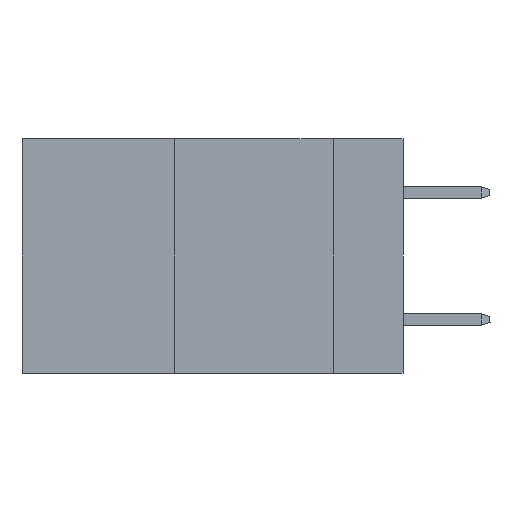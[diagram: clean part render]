
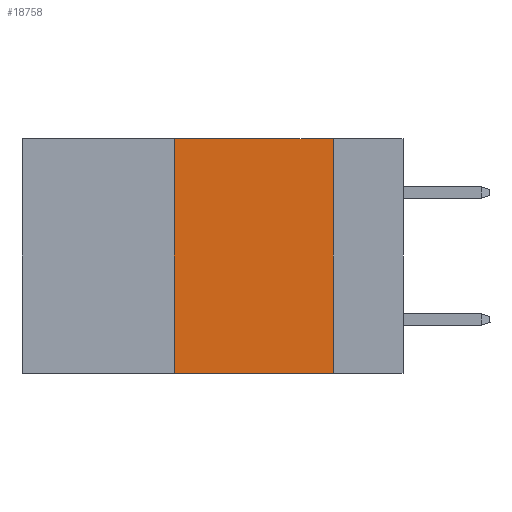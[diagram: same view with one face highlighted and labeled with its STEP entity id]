
A CAD part, left-side view. The second image highlights one B-rep face of the part: STEP entity #18758.
In plain terms, the highlighted planar face has unit normal (-1, 0, 0).
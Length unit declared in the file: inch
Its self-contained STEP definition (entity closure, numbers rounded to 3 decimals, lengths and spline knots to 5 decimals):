
#2084 = VERTEX_POINT ( 'NONE', #18589 ) ;
#2657 = LINE ( 'NONE', #15431, #31532 ) ;
#2737 = VERTEX_POINT ( 'NONE', #8233 ) ;
#3183 = DIRECTION ( 'NONE',  ( 0., 0., -1. ) ) ;
#3955 = DIRECTION ( 'NONE',  ( 0., -1., 0. ) ) ;
#4764 = AXIS2_PLACEMENT_3D ( 'NONE', #30969, #25291, #20306 ) ;
#8233 = CARTESIAN_POINT ( 'NONE',  ( 0., 0.36, 0. ) ) ;
#8951 = VECTOR ( 'NONE', #9687, 39.37008 ) ;
#8992 = CARTESIAN_POINT ( 'NONE',  ( 0., 0.36, -0.37 ) ) ;
#9687 = DIRECTION ( 'NONE',  ( 0., -1., 0. ) ) ;
#9983 = VECTOR ( 'NONE', #3183, 39.37008 ) ;
#10035 = FACE_OUTER_BOUND ( 'NONE', #23592, .T. ) ;
#12499 = ORIENTED_EDGE ( 'NONE', *, *, #22464, .F. ) ;
#12873 = DIRECTION ( 'NONE',  ( 0., 0., 1. ) ) ;
#13280 = ORIENTED_EDGE ( 'NONE', *, *, #28120, .F. ) ;
#15431 = CARTESIAN_POINT ( 'NONE',  ( 0., 0.36, 0. ) ) ;
#16124 = LINE ( 'NONE', #26617, #9983 ) ;
#16778 = LINE ( 'NONE', #27406, #31529 ) ;
#16931 = ORIENTED_EDGE ( 'NONE', *, *, #25445, .T. ) ;
#18466 = EDGE_CURVE ( 'NONE', #33410, #2737, #2657, .T. ) ;
#18589 = CARTESIAN_POINT ( 'NONE',  ( 0., 0.11, 0. ) ) ;
#18758 = ADVANCED_FACE ( 'NONE', ( #10035 ), #22745, .F. ) ;
#20306 = DIRECTION ( 'NONE',  ( 0., 0., -1. ) ) ;
#20839 = CARTESIAN_POINT ( 'NONE',  ( 0., 0.11, -0.37 ) ) ;
#21316 = VERTEX_POINT ( 'NONE', #20839 ) ;
#22464 = EDGE_CURVE ( 'NONE', #2084, #21316, #16124, .T. ) ;
#22715 = LINE ( 'NONE', #33177, #8951 ) ;
#22745 = PLANE ( 'NONE',  #4764 ) ;
#23592 = EDGE_LOOP ( 'NONE', ( #12499, #13280, #27113, #16931 ) ) ;
#25291 = DIRECTION ( 'NONE',  ( 1., 0., 0. ) ) ;
#25445 = EDGE_CURVE ( 'NONE', #33410, #21316, #22715, .T. ) ;
#26617 = CARTESIAN_POINT ( 'NONE',  ( 0., 0.11, 0. ) ) ;
#27113 = ORIENTED_EDGE ( 'NONE', *, *, #18466, .F. ) ;
#27406 = CARTESIAN_POINT ( 'NONE',  ( 0., 0.6, 0. ) ) ;
#28120 = EDGE_CURVE ( 'NONE', #2737, #2084, #16778, .T. ) ;
#30969 = CARTESIAN_POINT ( 'NONE',  ( 0., 0.6, 0. ) ) ;
#31529 = VECTOR ( 'NONE', #3955, 39.37008 ) ;
#31532 = VECTOR ( 'NONE', #12873, 39.37008 ) ;
#33177 = CARTESIAN_POINT ( 'NONE',  ( 0., 0.6, -0.37 ) ) ;
#33410 = VERTEX_POINT ( 'NONE', #8992 ) ;
